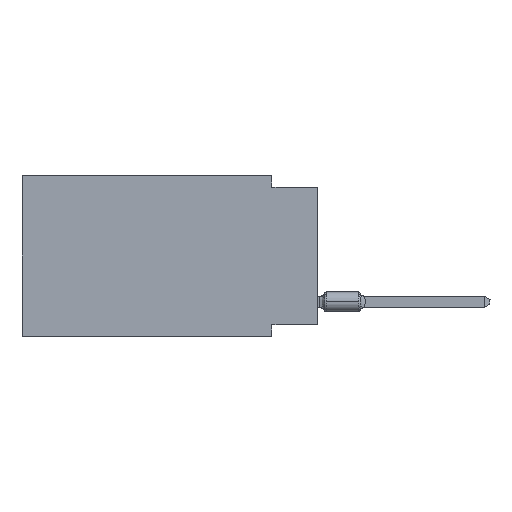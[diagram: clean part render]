
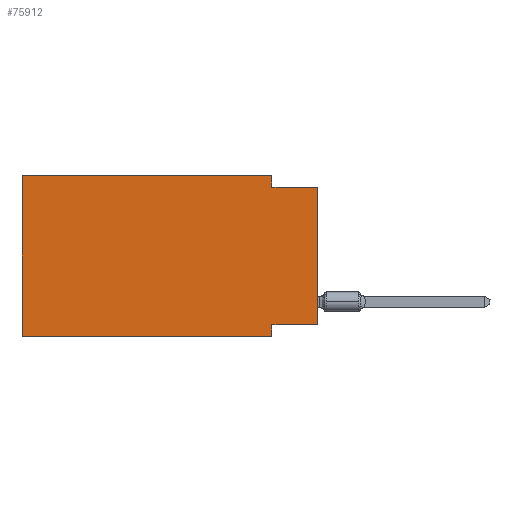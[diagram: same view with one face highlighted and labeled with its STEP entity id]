
A CAD part, left-side view. The second image highlights one B-rep face of the part: STEP entity #75912.
In plain terms, the highlighted planar face has unit normal (-1, 0, 0).
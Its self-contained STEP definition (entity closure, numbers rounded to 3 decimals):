
#4381 = VERTEX_POINT ( 'NONE', #59212 ) ;
#4571 = VERTEX_POINT ( 'NONE', #72142 ) ;
#5809 = LINE ( 'NONE', #113409, #112977 ) ;
#7164 = VERTEX_POINT ( 'NONE', #79890 ) ;
#9516 = ORIENTED_EDGE ( 'NONE', *, *, #25619, .T. ) ;
#10084 = DIRECTION ( 'NONE',  ( 0., 1., 0. ) ) ;
#12829 = AXIS2_PLACEMENT_3D ( 'NONE', #87359, #25624, #95588 ) ;
#13222 = DIRECTION ( 'NONE',  ( 0., -1., 0. ) ) ;
#14766 = DIRECTION ( 'NONE',  ( 0., 0., -1. ) ) ;
#17393 = CARTESIAN_POINT ( 'NONE',  ( 0., 0., 0. ) ) ;
#20308 = LINE ( 'NONE', #49078, #105242 ) ;
#20799 = EDGE_CURVE ( 'NONE', #22622, #112560, #53729, .T. ) ;
#22622 = VERTEX_POINT ( 'NONE', #55141 ) ;
#24633 = VECTOR ( 'NONE', #89602, 1000. ) ;
#25619 = EDGE_CURVE ( 'NONE', #22622, #57952, #20308, .T. ) ;
#25624 = DIRECTION ( 'NONE',  ( 1., 0., 0. ) ) ;
#32830 = DIRECTION ( 'NONE',  ( 0., -1., 0. ) ) ;
#34684 = DIRECTION ( 'NONE',  ( 0., 0., -1. ) ) ;
#34940 = ORIENTED_EDGE ( 'NONE', *, *, #113223, .F. ) ;
#36437 = CARTESIAN_POINT ( 'NONE',  ( 0., 2.54, -8.89 ) ) ;
#40558 = VECTOR ( 'NONE', #34684, 1000. ) ;
#40574 = ORIENTED_EDGE ( 'NONE', *, *, #41600, .F. ) ;
#41600 = EDGE_CURVE ( 'NONE', #4571, #4381, #92919, .T. ) ;
#44389 = LINE ( 'NONE', #44960, #105728 ) ;
#44960 = CARTESIAN_POINT ( 'NONE',  ( 0., 0., -0.635 ) ) ;
#45484 = CARTESIAN_POINT ( 'NONE',  ( 0., 16.383, 0. ) ) ;
#49078 = CARTESIAN_POINT ( 'NONE',  ( 0., 16.383, -8.89 ) ) ;
#53729 = LINE ( 'NONE', #45484, #24633 ) ;
#55141 = CARTESIAN_POINT ( 'NONE',  ( 0., 16.383, -8.89 ) ) ;
#56135 = VECTOR ( 'NONE', #107349, 1000. ) ;
#57952 = VERTEX_POINT ( 'NONE', #76525 ) ;
#59212 = CARTESIAN_POINT ( 'NONE',  ( 0., 2.54, -8.255 ) ) ;
#68227 = CARTESIAN_POINT ( 'NONE',  ( 0., 2.54, 0. ) ) ;
#69706 = EDGE_LOOP ( 'NONE', ( #71411, #88153, #92332, #108795, #84677, #9516, #34940, #40574 ) ) ;
#70302 = FACE_OUTER_BOUND ( 'NONE', #69706, .T. ) ;
#70803 = VERTEX_POINT ( 'NONE', #87946 ) ;
#71411 = ORIENTED_EDGE ( 'NONE', *, *, #75991, .T. ) ;
#71476 = LINE ( 'NONE', #17393, #56135 ) ;
#72142 = CARTESIAN_POINT ( 'NONE',  ( 0., 0., -8.255 ) ) ;
#75912 = ADVANCED_FACE ( 'NONE', ( #70302 ), #104430, .F. ) ;
#75991 = EDGE_CURVE ( 'NONE', #4571, #70803, #71476, .T. ) ;
#76525 = CARTESIAN_POINT ( 'NONE',  ( 0., 2.54, -8.89 ) ) ;
#79318 = EDGE_CURVE ( 'NONE', #7164, #70803, #44389, .T. ) ;
#79890 = CARTESIAN_POINT ( 'NONE',  ( 0., 2.54, -0.635 ) ) ;
#81135 = LINE ( 'NONE', #36437, #40558 ) ;
#83538 = VECTOR ( 'NONE', #10084, 1000. ) ;
#84677 = ORIENTED_EDGE ( 'NONE', *, *, #20799, .F. ) ;
#87359 = CARTESIAN_POINT ( 'NONE',  ( 0., 16.383, 0. ) ) ;
#87946 = CARTESIAN_POINT ( 'NONE',  ( 0., 0., -0.635 ) ) ;
#88153 = ORIENTED_EDGE ( 'NONE', *, *, #79318, .F. ) ;
#88218 = VECTOR ( 'NONE', #14766, 1000. ) ;
#89602 = DIRECTION ( 'NONE',  ( 0., 0., 1. ) ) ;
#90381 = CARTESIAN_POINT ( 'NONE',  ( 0., 16.383, 0. ) ) ;
#90636 = CARTESIAN_POINT ( 'NONE',  ( 0., 0., -8.255 ) ) ;
#92332 = ORIENTED_EDGE ( 'NONE', *, *, #116079, .F. ) ;
#92919 = LINE ( 'NONE', #90636, #83538 ) ;
#95588 = DIRECTION ( 'NONE',  ( 0., 0., -1. ) ) ;
#99879 = EDGE_CURVE ( 'NONE', #112560, #113054, #5809, .T. ) ;
#104137 = LINE ( 'NONE', #111235, #88218 ) ;
#104430 = PLANE ( 'NONE',  #12829 ) ;
#105242 = VECTOR ( 'NONE', #13222, 1000. ) ;
#105728 = VECTOR ( 'NONE', #115557, 1000. ) ;
#107349 = DIRECTION ( 'NONE',  ( 0., 0., 1. ) ) ;
#108795 = ORIENTED_EDGE ( 'NONE', *, *, #99879, .F. ) ;
#111235 = CARTESIAN_POINT ( 'NONE',  ( 0., 2.54, 0. ) ) ;
#112560 = VERTEX_POINT ( 'NONE', #90381 ) ;
#112977 = VECTOR ( 'NONE', #32830, 1000. ) ;
#113054 = VERTEX_POINT ( 'NONE', #68227 ) ;
#113223 = EDGE_CURVE ( 'NONE', #4381, #57952, #81135, .T. ) ;
#113409 = CARTESIAN_POINT ( 'NONE',  ( 0., 16.383, 0. ) ) ;
#115557 = DIRECTION ( 'NONE',  ( 0., -1., 0. ) ) ;
#116079 = EDGE_CURVE ( 'NONE', #113054, #7164, #104137, .T. ) ;
